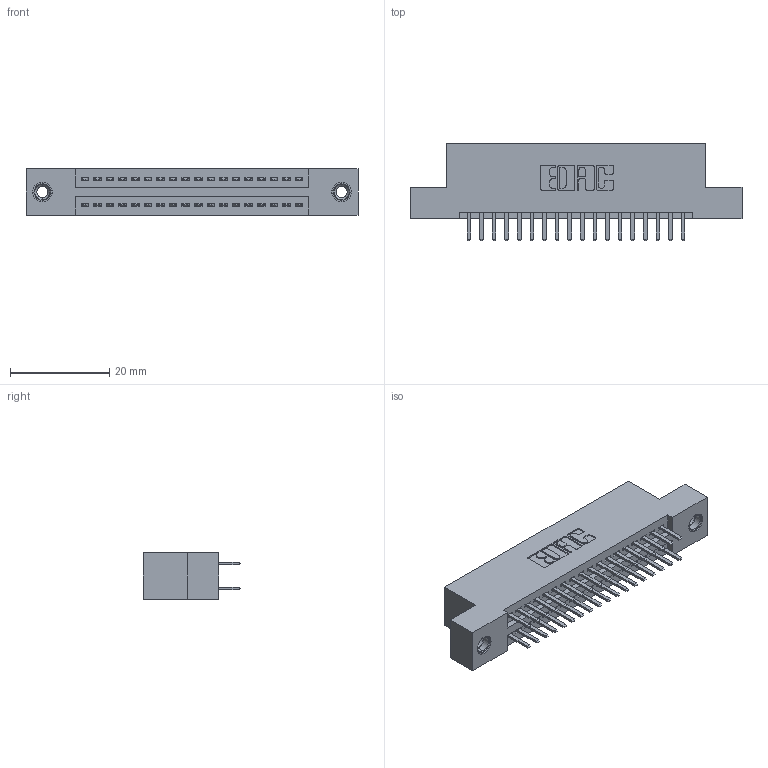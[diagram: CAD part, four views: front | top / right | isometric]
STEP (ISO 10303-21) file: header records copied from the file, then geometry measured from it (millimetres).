
FILE_DESCRIPTION (( 'STEP AP203' ), '1' );
FILE_NAME ('395-036-520-208.STEP', '2019-10-17T18:51:35', ( '' ), ( '' ), 'SwSTEP 2.0', 'SolidWorks 2016', '' );
FILE_SCHEMA (( 'CONFIG_CONTROL_DESIGN' ));
Length unit declared in the file: inch
Products named in the file (4): 345 Part_Flush Mounting Lugs - 0.156 Dia-TI; 345-292-001_345-293-120; 345-250-001_345-250-003-102; 395-036-520-208
Assembly tree (39 placements, depth 2):
  395-036-520-208
    345 Part_Flush Mounting Lugs - 0.156 Dia-TI
    345-292-001_345-293-120  x36
    345-250-001_345-250-003-102  x2
Bounding box: 66.93 x 19.68 x 9.4 mm (x, y, z)
Volume: 6256.4 mm3; surface area: 8763 mm2
Topology: 39 solids, 39 shells, 2130 faces, 6129 edges, 3982 vertices
Faces by surface type: plane 1372, cylinder 742, cone 12, torus 4
Entity records: 18654 total; most frequent: CARTESIAN_POINT 3143, ORIENTED_EDGE 3058, DIRECTION 2815, EDGE_CURVE 1529, VECTOR 1301, LINE 1301, VERTEX_POINT 1012, AXIS2_PLACEMENT_3D 757
